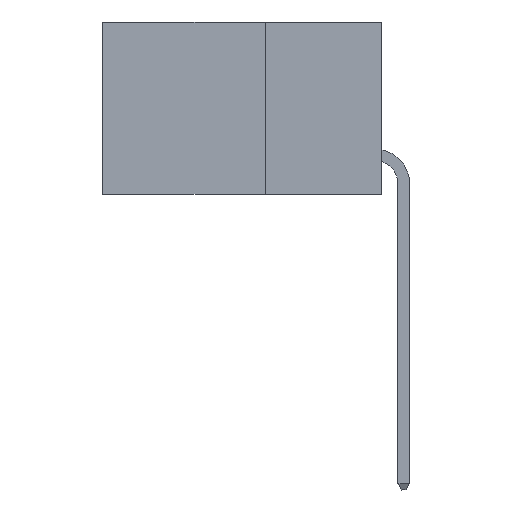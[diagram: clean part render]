
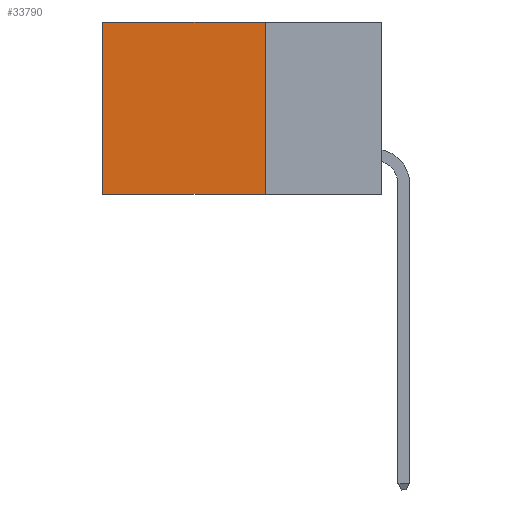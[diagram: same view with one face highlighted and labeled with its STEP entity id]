
A CAD part, left-side view. The second image highlights one B-rep face of the part: STEP entity #33790.
In plain terms, the highlighted planar face has unit normal (-1, 0, 0).
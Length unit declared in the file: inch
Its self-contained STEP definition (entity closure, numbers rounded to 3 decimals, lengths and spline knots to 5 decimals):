
#1097 = PLANE ( 'NONE',  #25958 ) ;
#1114 = CARTESIAN_POINT ( 'NONE',  ( 0.2875, 0.25, -0.37 ) ) ;
#1609 = DIRECTION ( 'NONE',  ( 0., 0., -1. ) ) ;
#4115 = DIRECTION ( 'NONE',  ( 1., 0., 0. ) ) ;
#4410 = CARTESIAN_POINT ( 'NONE',  ( 0.2875, 0.6, 0. ) ) ;
#6188 = LINE ( 'NONE', #4410, #28395 ) ;
#7998 = EDGE_CURVE ( 'NONE', #14133, #9505, #16991, .T. ) ;
#9505 = VERTEX_POINT ( 'NONE', #21170 ) ;
#10474 = CARTESIAN_POINT ( 'NONE',  ( 0.2875, 0.25, 0. ) ) ;
#11667 = VERTEX_POINT ( 'NONE', #10474 ) ;
#14133 = VERTEX_POINT ( 'NONE', #36715 ) ;
#14343 = LINE ( 'NONE', #35259, #29497 ) ;
#14990 = EDGE_LOOP ( 'NONE', ( #28454, #36538, #38221, #36104 ) ) ;
#15375 = LINE ( 'NONE', #19692, #31460 ) ;
#16991 = LINE ( 'NONE', #1114, #32127 ) ;
#17434 = CARTESIAN_POINT ( 'NONE',  ( 0.2875, 0.6, 0. ) ) ;
#19692 = CARTESIAN_POINT ( 'NONE',  ( 0.2875, 0.25, 0. ) ) ;
#20192 = DIRECTION ( 'NONE',  ( 0., 1., 0. ) ) ;
#21170 = CARTESIAN_POINT ( 'NONE',  ( 0.2875, 0.6, -0.37 ) ) ;
#21777 = EDGE_CURVE ( 'NONE', #25820, #9505, #6188, .T. ) ;
#22224 = CARTESIAN_POINT ( 'NONE',  ( 0.2875, 0.25, 0. ) ) ;
#22728 = FACE_OUTER_BOUND ( 'NONE', #14990, .T. ) ;
#25298 = DIRECTION ( 'NONE',  ( 0., 0., -1. ) ) ;
#25305 = DIRECTION ( 'NONE',  ( 0., 1., 0. ) ) ;
#25635 = EDGE_CURVE ( 'NONE', #11667, #14133, #15375, .T. ) ;
#25820 = VERTEX_POINT ( 'NONE', #17434 ) ;
#25958 = AXIS2_PLACEMENT_3D ( 'NONE', #22224, #4115, #25298 ) ;
#27454 = EDGE_CURVE ( 'NONE', #11667, #25820, #14343, .T. ) ;
#28395 = VECTOR ( 'NONE', #28615, 39.37008 ) ;
#28454 = ORIENTED_EDGE ( 'NONE', *, *, #21777, .T. ) ;
#28615 = DIRECTION ( 'NONE',  ( 0., 0., -1. ) ) ;
#29497 = VECTOR ( 'NONE', #20192, 39.37008 ) ;
#31460 = VECTOR ( 'NONE', #1609, 39.37008 ) ;
#32127 = VECTOR ( 'NONE', #25305, 39.37008 ) ;
#33790 = ADVANCED_FACE ( 'NONE', ( #22728 ), #1097, .F. ) ;
#35259 = CARTESIAN_POINT ( 'NONE',  ( 0.2875, 0.25, 0. ) ) ;
#36104 = ORIENTED_EDGE ( 'NONE', *, *, #27454, .T. ) ;
#36538 = ORIENTED_EDGE ( 'NONE', *, *, #7998, .F. ) ;
#36715 = CARTESIAN_POINT ( 'NONE',  ( 0.2875, 0.25, -0.37 ) ) ;
#38221 = ORIENTED_EDGE ( 'NONE', *, *, #25635, .F. ) ;
